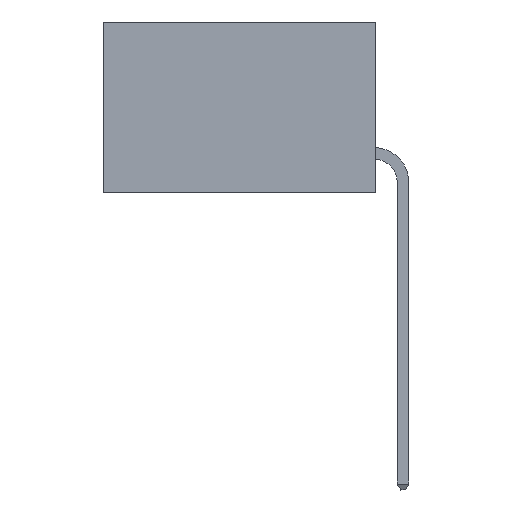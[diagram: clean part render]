
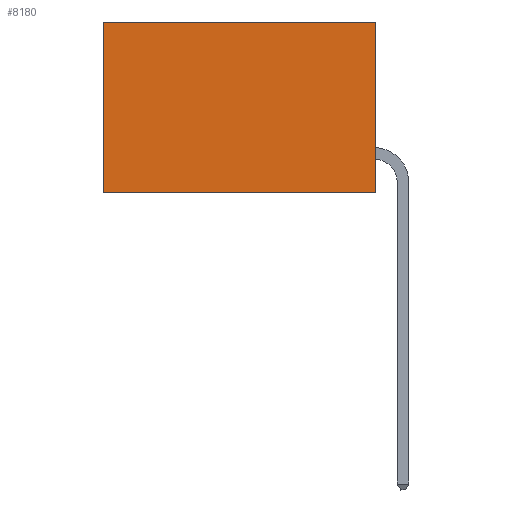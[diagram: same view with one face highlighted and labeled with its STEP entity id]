
A CAD part, left-side view. The second image highlights one B-rep face of the part: STEP entity #8180.
In plain terms, the highlighted planar face has unit normal (-1, 0, 0).
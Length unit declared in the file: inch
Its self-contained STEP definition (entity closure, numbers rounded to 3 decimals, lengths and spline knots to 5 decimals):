
#245 = CARTESIAN_POINT ( 'NONE',  ( 0.277, 0., -0.37 ) ) ;
#867 = ORIENTED_EDGE ( 'NONE', *, *, #4146, .T. ) ;
#1031 = DIRECTION ( 'NONE',  ( 0., 0., -1. ) ) ;
#1175 = VECTOR ( 'NONE', #2428, 39.37008 ) ;
#1277 = VECTOR ( 'NONE', #5932, 39.37008 ) ;
#1394 = EDGE_CURVE ( 'NONE', #8883, #5036, #5361, .T. ) ;
#1597 = CARTESIAN_POINT ( 'NONE',  ( 0.277, 0.59, -0.37 ) ) ;
#1695 = LINE ( 'NONE', #5773, #10115 ) ;
#2397 = VECTOR ( 'NONE', #10746, 39.37008 ) ;
#2428 = DIRECTION ( 'NONE',  ( 0., 1., 0. ) ) ;
#2449 = CARTESIAN_POINT ( 'NONE',  ( 0.277, 0., 0. ) ) ;
#3513 = FACE_OUTER_BOUND ( 'NONE', #9400, .T. ) ;
#3617 = ORIENTED_EDGE ( 'NONE', *, *, #8392, .F. ) ;
#4146 = EDGE_CURVE ( 'NONE', #11258, #8883, #9677, .T. ) ;
#4473 = PLANE ( 'NONE',  #6001 ) ;
#4974 = CARTESIAN_POINT ( 'NONE',  ( 0.277, 0., -0.37 ) ) ;
#5036 = VERTEX_POINT ( 'NONE', #12824 ) ;
#5361 = LINE ( 'NONE', #1597, #2397 ) ;
#5773 = CARTESIAN_POINT ( 'NONE',  ( 0.277, 0., -0.37 ) ) ;
#5932 = DIRECTION ( 'NONE',  ( 0., 1., 0. ) ) ;
#6001 = AXIS2_PLACEMENT_3D ( 'NONE', #11542, #7535, #1031 ) ;
#7535 = DIRECTION ( 'NONE',  ( 1., 0., 0. ) ) ;
#8180 = ADVANCED_FACE ( 'NONE', ( #3513 ), #4473, .F. ) ;
#8392 = EDGE_CURVE ( 'NONE', #11258, #13236, #1695, .T. ) ;
#8777 = ORIENTED_EDGE ( 'NONE', *, *, #1394, .T. ) ;
#8883 = VERTEX_POINT ( 'NONE', #10611 ) ;
#9400 = EDGE_LOOP ( 'NONE', ( #8777, #11446, #3617, #867 ) ) ;
#9677 = LINE ( 'NONE', #2449, #1175 ) ;
#10115 = VECTOR ( 'NONE', #11754, 39.37008 ) ;
#10436 = EDGE_CURVE ( 'NONE', #13236, #5036, #12109, .T. ) ;
#10611 = CARTESIAN_POINT ( 'NONE',  ( 0.277, 0.59, 0. ) ) ;
#10746 = DIRECTION ( 'NONE',  ( 0., 0., -1. ) ) ;
#11258 = VERTEX_POINT ( 'NONE', #12762 ) ;
#11446 = ORIENTED_EDGE ( 'NONE', *, *, #10436, .F. ) ;
#11542 = CARTESIAN_POINT ( 'NONE',  ( 0.277, 0., -0.37 ) ) ;
#11754 = DIRECTION ( 'NONE',  ( 0., 0., -1. ) ) ;
#12109 = LINE ( 'NONE', #245, #1277 ) ;
#12762 = CARTESIAN_POINT ( 'NONE',  ( 0.277, 0., 0. ) ) ;
#12824 = CARTESIAN_POINT ( 'NONE',  ( 0.277, 0.59, -0.37 ) ) ;
#13236 = VERTEX_POINT ( 'NONE', #4974 ) ;
